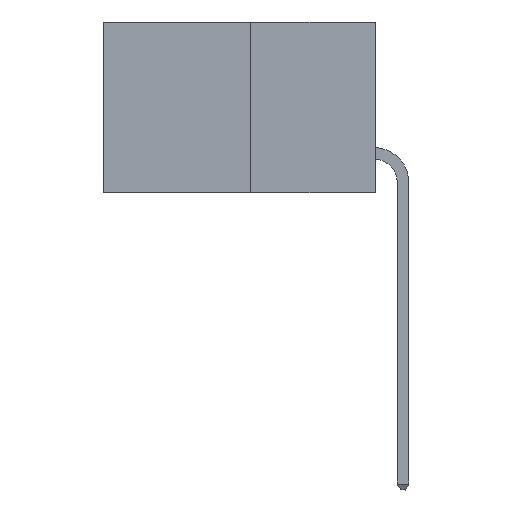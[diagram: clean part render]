
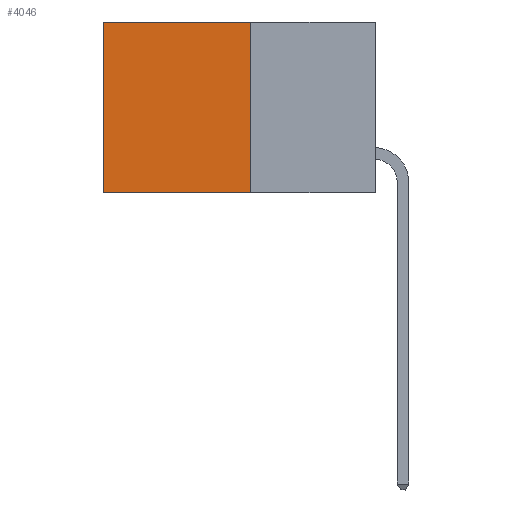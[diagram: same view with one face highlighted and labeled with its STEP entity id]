
A CAD part, left-side view. The second image highlights one B-rep face of the part: STEP entity #4046.
In plain terms, the highlighted planar face has unit normal (-1, 0, 0).
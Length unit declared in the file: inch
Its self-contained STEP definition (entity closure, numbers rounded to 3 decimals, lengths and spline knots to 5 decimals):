
#800 = CARTESIAN_POINT ( 'NONE',  ( 0.277, 0.59, -0.37 ) ) ;
#1004 = ORIENTED_EDGE ( 'NONE', *, *, #14875, .F. ) ;
#1161 = VERTEX_POINT ( 'NONE', #16683 ) ;
#1525 = ORIENTED_EDGE ( 'NONE', *, *, #3765, .F. ) ;
#1603 = VECTOR ( 'NONE', #9515, 39.37008 ) ;
#2084 = LINE ( 'NONE', #8069, #1603 ) ;
#2923 = DIRECTION ( 'NONE',  ( 1., 0., 0. ) ) ;
#3002 = VERTEX_POINT ( 'NONE', #10861 ) ;
#3765 = EDGE_CURVE ( 'NONE', #3002, #13045, #18906, .T. ) ;
#3912 = EDGE_CURVE ( 'NONE', #13134, #1161, #12348, .T. ) ;
#4046 = ADVANCED_FACE ( 'NONE', ( #9594 ), #17666, .F. ) ;
#6299 = CARTESIAN_POINT ( 'NONE',  ( 0.277, 0.27, -0.37 ) ) ;
#6407 = ORIENTED_EDGE ( 'NONE', *, *, #17068, .T. ) ;
#6680 = VECTOR ( 'NONE', #18008, 39.37008 ) ;
#7312 = VECTOR ( 'NONE', #16784, 39.37008 ) ;
#8019 = VECTOR ( 'NONE', #12797, 39.37008 ) ;
#8067 = CARTESIAN_POINT ( 'NONE',  ( 0.277, 0.27, -0.37 ) ) ;
#8069 = CARTESIAN_POINT ( 'NONE',  ( 0.277, 0.27, 0. ) ) ;
#9515 = DIRECTION ( 'NONE',  ( 0., 1., 0. ) ) ;
#9594 = FACE_OUTER_BOUND ( 'NONE', #11967, .T. ) ;
#10861 = CARTESIAN_POINT ( 'NONE',  ( 0.277, 0.27, 0. ) ) ;
#11874 = CARTESIAN_POINT ( 'NONE',  ( 0.277, 0.27, -0.37 ) ) ;
#11967 = EDGE_LOOP ( 'NONE', ( #14395, #1004, #1525, #6407 ) ) ;
#12256 = CARTESIAN_POINT ( 'NONE',  ( 0.277, 0.27, -0.37 ) ) ;
#12348 = LINE ( 'NONE', #800, #8019 ) ;
#12797 = DIRECTION ( 'NONE',  ( 0., 0., -1. ) ) ;
#13045 = VERTEX_POINT ( 'NONE', #12256 ) ;
#13134 = VERTEX_POINT ( 'NONE', #18254 ) ;
#13369 = DIRECTION ( 'NONE',  ( 0., 0., -1. ) ) ;
#13512 = AXIS2_PLACEMENT_3D ( 'NONE', #11874, #2923, #13369 ) ;
#14395 = ORIENTED_EDGE ( 'NONE', *, *, #3912, .T. ) ;
#14875 = EDGE_CURVE ( 'NONE', #13045, #1161, #18318, .T. ) ;
#16683 = CARTESIAN_POINT ( 'NONE',  ( 0.277, 0.59, -0.37 ) ) ;
#16784 = DIRECTION ( 'NONE',  ( 0., 0., -1. ) ) ;
#17068 = EDGE_CURVE ( 'NONE', #3002, #13134, #2084, .T. ) ;
#17666 = PLANE ( 'NONE',  #13512 ) ;
#18008 = DIRECTION ( 'NONE',  ( 0., 1., 0. ) ) ;
#18254 = CARTESIAN_POINT ( 'NONE',  ( 0.277, 0.59, 0. ) ) ;
#18318 = LINE ( 'NONE', #6299, #6680 ) ;
#18906 = LINE ( 'NONE', #8067, #7312 ) ;
